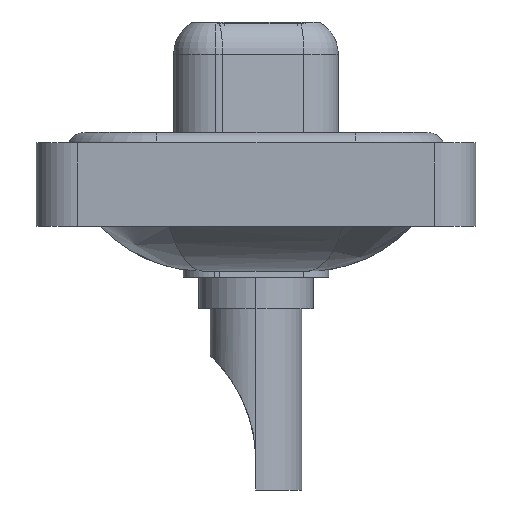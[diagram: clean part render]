
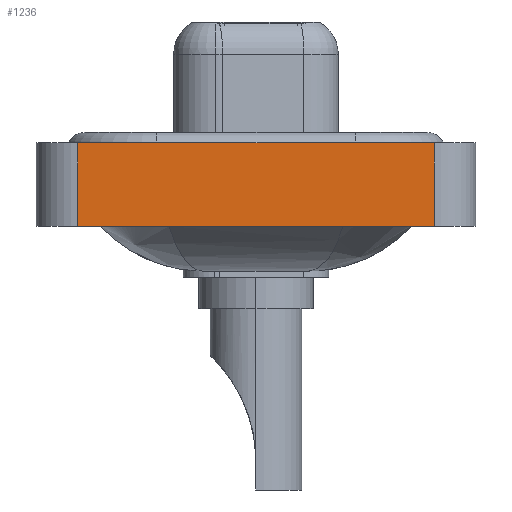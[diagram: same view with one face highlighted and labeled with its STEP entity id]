
A CAD part, left-side view. The second image highlights one B-rep face of the part: STEP entity #1236.
In plain terms, the highlighted planar face has unit normal (-1, 0, 0).
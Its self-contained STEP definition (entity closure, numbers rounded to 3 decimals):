
#337 = DIRECTION ( 'NONE',  ( 0., -1., 0. ) ) ;
#535 = VERTEX_POINT ( 'NONE', #14242 ) ;
#1236 = ADVANCED_FACE ( 'NONE', ( #16412 ), #13233, .T. ) ;
#1860 = EDGE_CURVE ( 'NONE', #535, #6061, #2243, .T. ) ;
#2243 = LINE ( 'NONE', #8668, #6842 ) ;
#2523 = CARTESIAN_POINT ( 'NONE',  ( -7.3, -8.55, 0.4 ) ) ;
#2797 = LINE ( 'NONE', #12919, #17666 ) ;
#3426 = VERTEX_POINT ( 'NONE', #15601 ) ;
#3570 = DIRECTION ( 'NONE',  ( 0., 0., 1. ) ) ;
#3879 = LINE ( 'NONE', #15066, #10252 ) ;
#4625 = CARTESIAN_POINT ( 'NONE',  ( -7.3, -8.55, -3.6 ) ) ;
#5211 = CARTESIAN_POINT ( 'NONE',  ( -7.3, -8.55, -3.6 ) ) ;
#6061 = VERTEX_POINT ( 'NONE', #2523 ) ;
#6101 = VECTOR ( 'NONE', #15372, 1000. ) ;
#6789 = DIRECTION ( 'NONE',  ( -1., 0., 0. ) ) ;
#6842 = VECTOR ( 'NONE', #7068, 1000. ) ;
#7068 = DIRECTION ( 'NONE',  ( 0., -1., 0. ) ) ;
#7227 = VERTEX_POINT ( 'NONE', #8059 ) ;
#7858 = AXIS2_PLACEMENT_3D ( 'NONE', #5211, #6789, #14537 ) ;
#8059 = CARTESIAN_POINT ( 'NONE',  ( -7.3, 8.55, -3.6 ) ) ;
#8668 = CARTESIAN_POINT ( 'NONE',  ( -7.3, -8.55, 0.4 ) ) ;
#9733 = EDGE_CURVE ( 'NONE', #7227, #535, #3879, .T. ) ;
#10252 = VECTOR ( 'NONE', #3570, 1000. ) ;
#10813 = ORIENTED_EDGE ( 'NONE', *, *, #9733, .F. ) ;
#12626 = LINE ( 'NONE', #4625, #6101 ) ;
#12919 = CARTESIAN_POINT ( 'NONE',  ( -7.3, -8.55, -3.6 ) ) ;
#13233 = PLANE ( 'NONE',  #7858 ) ;
#14242 = CARTESIAN_POINT ( 'NONE',  ( -7.3, 8.55, 0.4 ) ) ;
#14537 = DIRECTION ( 'NONE',  ( 0., 0., 1. ) ) ;
#14601 = EDGE_CURVE ( 'NONE', #7227, #3426, #2797, .T. ) ;
#14752 = EDGE_LOOP ( 'NONE', ( #18492, #19918, #10813, #17885 ) ) ;
#15066 = CARTESIAN_POINT ( 'NONE',  ( -7.3, 8.55, -3.6 ) ) ;
#15372 = DIRECTION ( 'NONE',  ( 0., 0., 1. ) ) ;
#15601 = CARTESIAN_POINT ( 'NONE',  ( -7.3, -8.55, -3.6 ) ) ;
#15946 = EDGE_CURVE ( 'NONE', #3426, #6061, #12626, .T. ) ;
#16412 = FACE_OUTER_BOUND ( 'NONE', #14752, .T. ) ;
#17666 = VECTOR ( 'NONE', #337, 1000. ) ;
#17885 = ORIENTED_EDGE ( 'NONE', *, *, #14601, .T. ) ;
#18492 = ORIENTED_EDGE ( 'NONE', *, *, #15946, .T. ) ;
#19918 = ORIENTED_EDGE ( 'NONE', *, *, #1860, .F. ) ;
